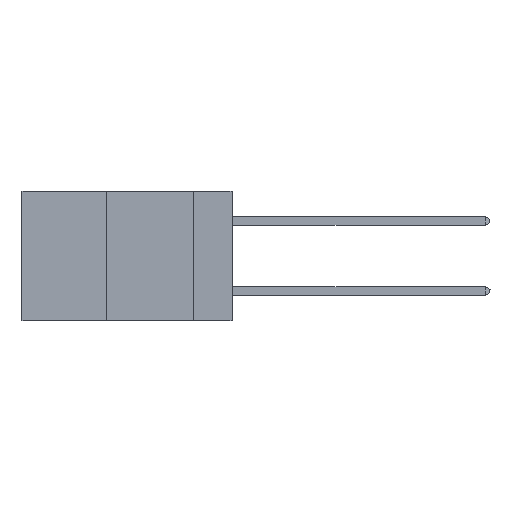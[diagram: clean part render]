
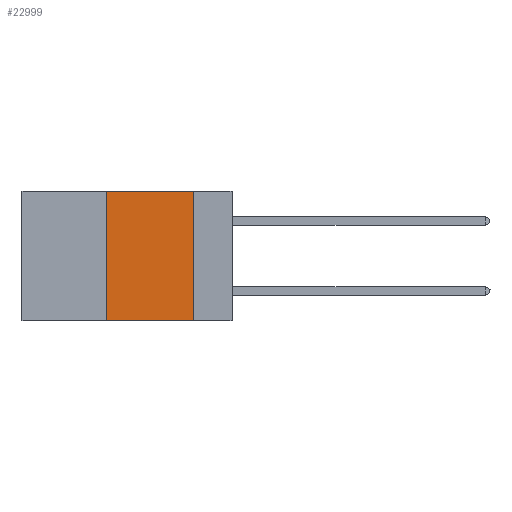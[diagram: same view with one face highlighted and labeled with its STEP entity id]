
A CAD part, left-side view. The second image highlights one B-rep face of the part: STEP entity #22999.
In plain terms, the highlighted planar face has unit normal (-1, 0, 0).
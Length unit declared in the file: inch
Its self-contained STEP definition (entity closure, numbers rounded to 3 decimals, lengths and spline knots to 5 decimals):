
#1068 = VECTOR ( 'NONE', #5579, 39.37008 ) ;
#1151 = VERTEX_POINT ( 'NONE', #12871 ) ;
#1796 = CARTESIAN_POINT ( 'NONE',  ( 0., 0.36, 0. ) ) ;
#3092 = ORIENTED_EDGE ( 'NONE', *, *, #22415, .T. ) ;
#3604 = VERTEX_POINT ( 'NONE', #5376 ) ;
#3628 = AXIS2_PLACEMENT_3D ( 'NONE', #23040, #5389, #19603 ) ;
#4715 = LINE ( 'NONE', #18993, #9971 ) ;
#5376 = CARTESIAN_POINT ( 'NONE',  ( 0., 0.11, -0.37 ) ) ;
#5389 = DIRECTION ( 'NONE',  ( 1., 0., 0. ) ) ;
#5579 = DIRECTION ( 'NONE',  ( 0., -1., 0. ) ) ;
#6577 = VECTOR ( 'NONE', #14264, 39.37008 ) ;
#6861 = LINE ( 'NONE', #1796, #6577 ) ;
#8217 = VERTEX_POINT ( 'NONE', #19399 ) ;
#9371 = LINE ( 'NONE', #13251, #21918 ) ;
#9965 = CARTESIAN_POINT ( 'NONE',  ( 0., 0.36, 0. ) ) ;
#9971 = VECTOR ( 'NONE', #10209, 39.37008 ) ;
#10209 = DIRECTION ( 'NONE',  ( 0., -1., 0. ) ) ;
#10521 = ORIENTED_EDGE ( 'NONE', *, *, #14727, .F. ) ;
#12871 = CARTESIAN_POINT ( 'NONE',  ( 0., 0.11, 0. ) ) ;
#13251 = CARTESIAN_POINT ( 'NONE',  ( 0., 0.11, 0. ) ) ;
#14188 = VERTEX_POINT ( 'NONE', #9965 ) ;
#14264 = DIRECTION ( 'NONE',  ( 0., 0., 1. ) ) ;
#14270 = EDGE_CURVE ( 'NONE', #14188, #1151, #4715, .T. ) ;
#14727 = EDGE_CURVE ( 'NONE', #1151, #3604, #9371, .T. ) ;
#15503 = ORIENTED_EDGE ( 'NONE', *, *, #14270, .F. ) ;
#16700 = DIRECTION ( 'NONE',  ( 0., 0., -1. ) ) ;
#18421 = FACE_OUTER_BOUND ( 'NONE', #20577, .T. ) ;
#18993 = CARTESIAN_POINT ( 'NONE',  ( 0., 0.6, 0. ) ) ;
#19278 = EDGE_CURVE ( 'NONE', #8217, #14188, #6861, .T. ) ;
#19399 = CARTESIAN_POINT ( 'NONE',  ( 0., 0.36, -0.37 ) ) ;
#19543 = LINE ( 'NONE', #21724, #1068 ) ;
#19603 = DIRECTION ( 'NONE',  ( 0., 0., -1. ) ) ;
#20079 = ORIENTED_EDGE ( 'NONE', *, *, #19278, .F. ) ;
#20577 = EDGE_LOOP ( 'NONE', ( #10521, #15503, #20079, #3092 ) ) ;
#21295 = PLANE ( 'NONE',  #3628 ) ;
#21724 = CARTESIAN_POINT ( 'NONE',  ( 0., 0.6, -0.37 ) ) ;
#21918 = VECTOR ( 'NONE', #16700, 39.37008 ) ;
#22415 = EDGE_CURVE ( 'NONE', #8217, #3604, #19543, .T. ) ;
#22999 = ADVANCED_FACE ( 'NONE', ( #18421 ), #21295, .F. ) ;
#23040 = CARTESIAN_POINT ( 'NONE',  ( 0., 0.6, 0. ) ) ;
